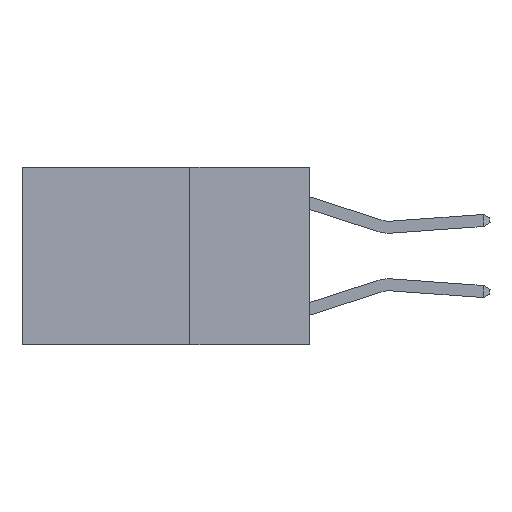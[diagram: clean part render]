
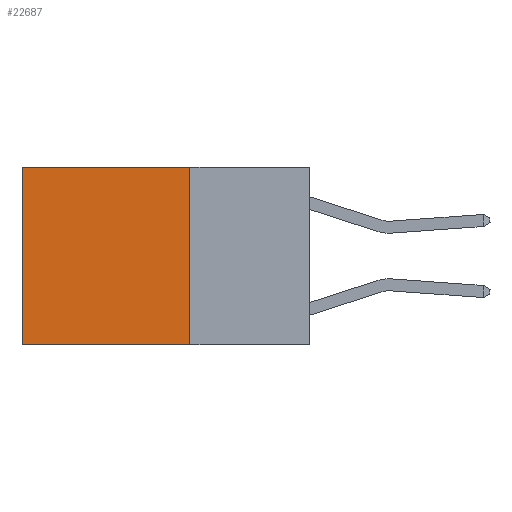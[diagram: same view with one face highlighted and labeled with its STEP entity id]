
A CAD part, left-side view. The second image highlights one B-rep face of the part: STEP entity #22687.
In plain terms, the highlighted planar face has unit normal (-1, 0, 0).
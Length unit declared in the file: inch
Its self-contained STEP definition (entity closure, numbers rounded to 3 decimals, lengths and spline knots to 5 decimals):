
#527 = ORIENTED_EDGE ( 'NONE', *, *, #6785, .T. ) ;
#1538 = CARTESIAN_POINT ( 'NONE',  ( 0.2625, 0.25, 0. ) ) ;
#2007 = VECTOR ( 'NONE', #17327, 39.37008 ) ;
#2015 = AXIS2_PLACEMENT_3D ( 'NONE', #1538, #16565, #5257 ) ;
#2157 = DIRECTION ( 'NONE',  ( 0., 1., 0. ) ) ;
#2364 = VECTOR ( 'NONE', #2157, 39.37008 ) ;
#2380 = EDGE_CURVE ( 'NONE', #17488, #6935, #5795, .T. ) ;
#2953 = CARTESIAN_POINT ( 'NONE',  ( 0.2625, 0.6, -0.37 ) ) ;
#3558 = ORIENTED_EDGE ( 'NONE', *, *, #5582, .T. ) ;
#3743 = CARTESIAN_POINT ( 'NONE',  ( 0.2625, 0.6, 0. ) ) ;
#4398 = LINE ( 'NONE', #8374, #2007 ) ;
#5257 = DIRECTION ( 'NONE',  ( 0., 0., -1. ) ) ;
#5582 = EDGE_CURVE ( 'NONE', #17488, #19890, #7885, .T. ) ;
#5795 = LINE ( 'NONE', #13357, #9661 ) ;
#6356 = DIRECTION ( 'NONE',  ( 0., 1., 0. ) ) ;
#6785 = EDGE_CURVE ( 'NONE', #19890, #21850, #4398, .T. ) ;
#6935 = VERTEX_POINT ( 'NONE', #21951 ) ;
#7012 = PLANE ( 'NONE',  #2015 ) ;
#7499 = FACE_OUTER_BOUND ( 'NONE', #11817, .T. ) ;
#7534 = LINE ( 'NONE', #15674, #15616 ) ;
#7885 = LINE ( 'NONE', #13818, #2364 ) ;
#8374 = CARTESIAN_POINT ( 'NONE',  ( 0.2625, 0.6, 0. ) ) ;
#8800 = EDGE_CURVE ( 'NONE', #6935, #21850, #7534, .T. ) ;
#9661 = VECTOR ( 'NONE', #21003, 39.37008 ) ;
#11817 = EDGE_LOOP ( 'NONE', ( #527, #16150, #12215, #3558 ) ) ;
#12215 = ORIENTED_EDGE ( 'NONE', *, *, #2380, .F. ) ;
#13357 = CARTESIAN_POINT ( 'NONE',  ( 0.2625, 0.25, 0. ) ) ;
#13818 = CARTESIAN_POINT ( 'NONE',  ( 0.2625, 0.25, 0. ) ) ;
#15616 = VECTOR ( 'NONE', #6356, 39.37008 ) ;
#15674 = CARTESIAN_POINT ( 'NONE',  ( 0.2625, 0.25, -0.37 ) ) ;
#16150 = ORIENTED_EDGE ( 'NONE', *, *, #8800, .F. ) ;
#16565 = DIRECTION ( 'NONE',  ( 1., 0., 0. ) ) ;
#17327 = DIRECTION ( 'NONE',  ( 0., 0., -1. ) ) ;
#17488 = VERTEX_POINT ( 'NONE', #20460 ) ;
#19890 = VERTEX_POINT ( 'NONE', #3743 ) ;
#20460 = CARTESIAN_POINT ( 'NONE',  ( 0.2625, 0.25, 0. ) ) ;
#21003 = DIRECTION ( 'NONE',  ( 0., 0., -1. ) ) ;
#21850 = VERTEX_POINT ( 'NONE', #2953 ) ;
#21951 = CARTESIAN_POINT ( 'NONE',  ( 0.2625, 0.25, -0.37 ) ) ;
#22687 = ADVANCED_FACE ( 'NONE', ( #7499 ), #7012, .F. ) ;
